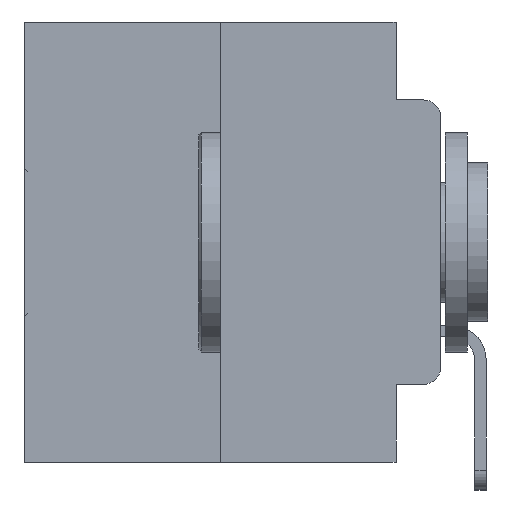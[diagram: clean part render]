
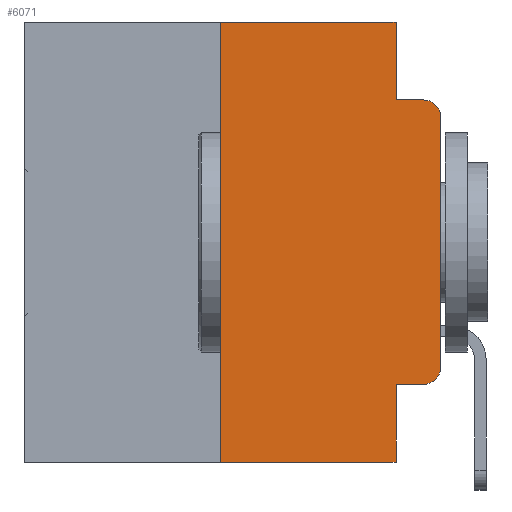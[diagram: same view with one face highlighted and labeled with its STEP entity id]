
A CAD part, left-side view. The second image highlights one B-rep face of the part: STEP entity #6071.
In plain terms, the highlighted planar face has unit normal (-1, 0, 0).
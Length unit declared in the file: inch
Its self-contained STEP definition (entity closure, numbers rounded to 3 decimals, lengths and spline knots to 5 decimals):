
#52 = DIRECTION ( 'NONE',  ( -1., 0., 0. ) ) ;
#517 = EDGE_CURVE ( 'NONE', #10914, #8589, #13361, .T. ) ;
#1320 = VERTEX_POINT ( 'NONE', #25461 ) ;
#1645 = ORIENTED_EDGE ( 'NONE', *, *, #29699, .F. ) ;
#1713 = LINE ( 'NONE', #30013, #26008 ) ;
#2117 = ORIENTED_EDGE ( 'NONE', *, *, #9147, .F. ) ;
#2989 = ORIENTED_EDGE ( 'NONE', *, *, #9501, .F. ) ;
#3323 = ORIENTED_EDGE ( 'NONE', *, *, #8913, .F. ) ;
#3959 = VECTOR ( 'NONE', #28896, 39.37008 ) ;
#4094 = EDGE_CURVE ( 'NONE', #22735, #17808, #15747, .T. ) ;
#4193 = DIRECTION ( 'NONE',  ( 0., 0., 1. ) ) ;
#4225 = ORIENTED_EDGE ( 'NONE', *, *, #29456, .T. ) ;
#4713 = ORIENTED_EDGE ( 'NONE', *, *, #4094, .F. ) ;
#4861 = CARTESIAN_POINT ( 'NONE',  ( 0., 0.051, -0.0885 ) ) ;
#5109 = EDGE_CURVE ( 'NONE', #21293, #10751, #17170, .T. ) ;
#5122 = ORIENTED_EDGE ( 'NONE', *, *, #8591, .T. ) ;
#5598 = DIRECTION ( 'NONE',  ( 1., 0., 0. ) ) ;
#5727 = VECTOR ( 'NONE', #10694, 39.37008 ) ;
#5995 = CARTESIAN_POINT ( 'NONE',  ( 0., 0.25, 0. ) ) ;
#6020 = DIRECTION ( 'NONE',  ( 0., -1., 0. ) ) ;
#6071 = ADVANCED_FACE ( 'NONE', ( #29335 ), #28836, .F. ) ;
#7290 = CARTESIAN_POINT ( 'NONE',  ( 0., 0.02, -0.4115 ) ) ;
#7777 = CARTESIAN_POINT ( 'NONE',  ( 0., 0.051, 0. ) ) ;
#8589 = VERTEX_POINT ( 'NONE', #7290 ) ;
#8591 = EDGE_CURVE ( 'NONE', #8589, #21293, #16937, .T. ) ;
#8651 = CARTESIAN_POINT ( 'NONE',  ( 0., 0., -0.1085 ) ) ;
#8900 = CARTESIAN_POINT ( 'NONE',  ( 0., 0., 0. ) ) ;
#8913 = EDGE_CURVE ( 'NONE', #17808, #22599, #26690, .T. ) ;
#8985 = VERTEX_POINT ( 'NONE', #20303 ) ;
#9083 = CARTESIAN_POINT ( 'NONE',  ( 0., 0.02, -0.1085 ) ) ;
#9147 = EDGE_CURVE ( 'NONE', #1320, #22735, #1713, .T. ) ;
#9242 = DIRECTION ( 'NONE',  ( 0., -1., 0. ) ) ;
#9501 = EDGE_CURVE ( 'NONE', #10914, #8985, #23412, .T. ) ;
#9776 = ORIENTED_EDGE ( 'NONE', *, *, #517, .T. ) ;
#9849 = CARTESIAN_POINT ( 'NONE',  ( 0., 0.473, -0.5 ) ) ;
#9879 = ORIENTED_EDGE ( 'NONE', *, *, #22981, .T. ) ;
#10694 = DIRECTION ( 'NONE',  ( 0., 0., 1. ) ) ;
#10751 = VERTEX_POINT ( 'NONE', #8651 ) ;
#10914 = VERTEX_POINT ( 'NONE', #20824 ) ;
#11493 = DIRECTION ( 'NONE',  ( 0., 0., -1. ) ) ;
#12255 = DIRECTION ( 'NONE',  ( 0., -1., 0. ) ) ;
#13086 = VERTEX_POINT ( 'NONE', #20149 ) ;
#13164 = LINE ( 'NONE', #9849, #24767 ) ;
#13361 = LINE ( 'NONE', #21358, #29604 ) ;
#13523 = LINE ( 'NONE', #5995, #5727 ) ;
#14153 = CIRCLE ( 'NONE', #18063, 0.02 ) ;
#14408 = CARTESIAN_POINT ( 'NONE',  ( 0., 0.02, -0.3915 ) ) ;
#15073 = VECTOR ( 'NONE', #6020, 39.37008 ) ;
#15225 = CARTESIAN_POINT ( 'NONE',  ( 0., 0., -0.3915 ) ) ;
#15747 = LINE ( 'NONE', #18011, #21900 ) ;
#16778 = DIRECTION ( 'NONE',  ( 0., 0., -1. ) ) ;
#16937 = CIRCLE ( 'NONE', #28990, 0.02 ) ;
#17170 = LINE ( 'NONE', #8900, #27985 ) ;
#17806 = CARTESIAN_POINT ( 'NONE',  ( 0., 0.051, -0.0885 ) ) ;
#17808 = VERTEX_POINT ( 'NONE', #4861 ) ;
#18011 = CARTESIAN_POINT ( 'NONE',  ( 0., 0.051, 0. ) ) ;
#18063 = AXIS2_PLACEMENT_3D ( 'NONE', #9083, #25391, #11493 ) ;
#19702 = CARTESIAN_POINT ( 'NONE',  ( 0., 0.473, 0. ) ) ;
#19782 = CARTESIAN_POINT ( 'NONE',  ( 0., 0.051, 0. ) ) ;
#20149 = CARTESIAN_POINT ( 'NONE',  ( 0., 0.25, -0.5 ) ) ;
#20303 = CARTESIAN_POINT ( 'NONE',  ( 0., 0.051, -0.5 ) ) ;
#20824 = CARTESIAN_POINT ( 'NONE',  ( 0., 0.051, -0.4115 ) ) ;
#21293 = VERTEX_POINT ( 'NONE', #15225 ) ;
#21358 = CARTESIAN_POINT ( 'NONE',  ( 0., 0.051, -0.4115 ) ) ;
#21900 = VECTOR ( 'NONE', #29428, 39.37008 ) ;
#22008 = DIRECTION ( 'NONE',  ( 0., 0., -1. ) ) ;
#22599 = VERTEX_POINT ( 'NONE', #26070 ) ;
#22735 = VERTEX_POINT ( 'NONE', #7777 ) ;
#22981 = EDGE_CURVE ( 'NONE', #10751, #22599, #14153, .T. ) ;
#23412 = LINE ( 'NONE', #19782, #3959 ) ;
#23547 = ORIENTED_EDGE ( 'NONE', *, *, #5109, .T. ) ;
#24767 = VECTOR ( 'NONE', #12255, 39.37008 ) ;
#25391 = DIRECTION ( 'NONE',  ( -1., 0., 0. ) ) ;
#25461 = CARTESIAN_POINT ( 'NONE',  ( 0., 0.25, 0. ) ) ;
#26008 = VECTOR ( 'NONE', #9242, 39.37008 ) ;
#26070 = CARTESIAN_POINT ( 'NONE',  ( 0., 0.02, -0.0885 ) ) ;
#26690 = LINE ( 'NONE', #17806, #15073 ) ;
#27471 = AXIS2_PLACEMENT_3D ( 'NONE', #19702, #5598, #22008 ) ;
#27985 = VECTOR ( 'NONE', #4193, 39.37008 ) ;
#28473 = EDGE_LOOP ( 'NONE', ( #23547, #9879, #3323, #4713, #2117, #1645, #4225, #2989, #9776, #5122 ) ) ;
#28836 = PLANE ( 'NONE',  #27471 ) ;
#28896 = DIRECTION ( 'NONE',  ( 0., 0., -1. ) ) ;
#28990 = AXIS2_PLACEMENT_3D ( 'NONE', #14408, #52, #16778 ) ;
#29335 = FACE_OUTER_BOUND ( 'NONE', #28473, .T. ) ;
#29428 = DIRECTION ( 'NONE',  ( 0., 0., -1. ) ) ;
#29456 = EDGE_CURVE ( 'NONE', #13086, #8985, #13164, .T. ) ;
#29604 = VECTOR ( 'NONE', #29664, 39.37008 ) ;
#29664 = DIRECTION ( 'NONE',  ( 0., -1., 0. ) ) ;
#29699 = EDGE_CURVE ( 'NONE', #13086, #1320, #13523, .T. ) ;
#30013 = CARTESIAN_POINT ( 'NONE',  ( 0., 0.473, 0. ) ) ;
